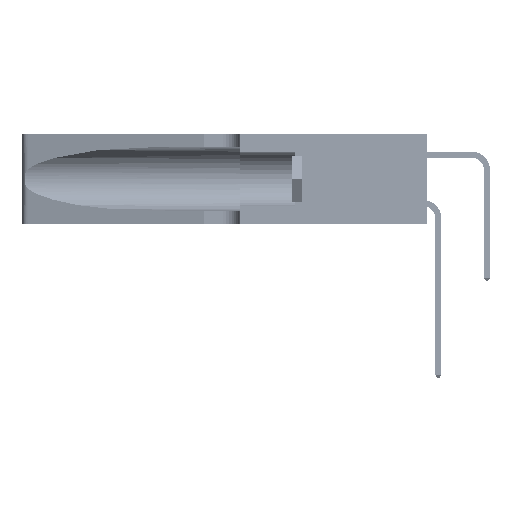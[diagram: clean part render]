
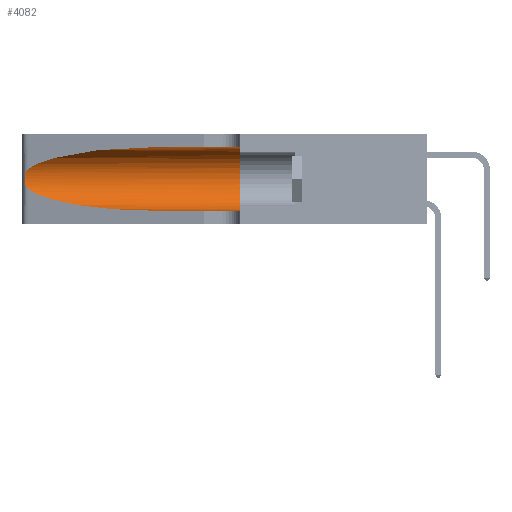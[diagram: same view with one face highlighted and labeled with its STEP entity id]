
A CAD part, left-side view. The second image highlights one B-rep face of the part: STEP entity #4082.
In plain terms, the highlighted cylindrical face has radius 3.308 mm (diameter 6.617 mm), a partial arc.
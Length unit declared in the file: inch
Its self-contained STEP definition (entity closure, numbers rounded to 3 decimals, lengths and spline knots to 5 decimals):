
#132 = LINE ( 'NONE', #53798, #2145 ) ;
#247 = CARTESIAN_POINT ( 'NONE',  ( 0.1305, 0.35, 0.185 ) ) ;
#2145 = VECTOR ( 'NONE', #22762, 39.37008 ) ;
#4082 = ADVANCED_FACE ( 'NONE', ( #48773 ), #19457, .F. ) ;
#4983 = VERTEX_POINT ( 'NONE', #8598 ) ;
#5031 = CIRCLE ( 'NONE', #31959, 0.13025 ) ;
#7638 = CARTESIAN_POINT ( 'NONE',  ( 0.25487, 1.22718, 0.22369 ) ) ;
#7841 = EDGE_CURVE ( 'NONE', #52570, #32961, #28715, .T. ) ;
#7964 = CARTESIAN_POINT ( 'NONE',  ( 0.1305, 0.72297, 0.05475 ) ) ;
#8035 = AXIS2_PLACEMENT_3D ( 'NONE', #45340, #50082, #14811 ) ;
#8598 = CARTESIAN_POINT ( 'NONE',  ( 0.1305, 0.35, 0.31525 ) ) ;
#8722 = CARTESIAN_POINT ( 'NONE',  ( 0.25789, 1.23486, 0.15765 ) ) ;
#9101 = CARTESIAN_POINT ( 'NONE',  ( 0.25555, 1.22994, 0.2215 ) ) ;
#11456 = ORIENTED_EDGE ( 'NONE', *, *, #47455, .F. ) ;
#12190 = CARTESIAN_POINT ( 'NONE',  ( 0.25487, 1.22718, 0.14631 ) ) ;
#13143 = CARTESIAN_POINT ( 'NONE',  ( 0.25555, 1.22993, 0.14849 ) ) ;
#14784 = CARTESIAN_POINT ( 'NONE',  ( 0.1305, 0.72297, 0.05475 ) ) ;
#14811 = DIRECTION ( 'NONE',  ( 0., 0., -1. ) ) ;
#16566 = CARTESIAN_POINT ( 'NONE',  ( 0.18966, 0.96281, 0.05475 ) ) ;
#17701 = CARTESIAN_POINT ( 'NONE',  ( 0.26018, 1.23835, 0.19895 ) ) ;
#18547 = ORIENTED_EDGE ( 'NONE', *, *, #20131, .F. ) ;
#19457 = CYLINDRICAL_SURFACE ( 'NONE', #8035, 0.13025 ) ;
#20131 = EDGE_CURVE ( 'NONE', #4983, #32767, #5031, .T. ) ;
#21354 = CARTESIAN_POINT ( 'NONE',  ( 0.26075, 1.23896, 0.178 ) ) ;
#21537 = CARTESIAN_POINT ( 'NONE',  ( 0.25487, 1.22718, 0.22369 ) ) ;
#22079 =( BOUNDED_CURVE ( )  B_SPLINE_CURVE ( 3, ( #42907, #56063, #25947, #7638 ),
 .UNSPECIFIED., .F., .F. ) 
 B_SPLINE_CURVE_WITH_KNOTS ( ( 4, 4 ),
 ( 1.5708, 2.84003 ),
 .UNSPECIFIED. ) 
 CURVE ( )  GEOMETRIC_REPRESENTATION_ITEM ( )  RATIONAL_B_SPLINE_CURVE ( ( 1., 0.87, 0.87, 1. ) ) 
 REPRESENTATION_ITEM ( '' )  );
#22762 = DIRECTION ( 'NONE',  ( 0., -1., 0. ) ) ;
#23532 = CARTESIAN_POINT ( 'NONE',  ( 0.25487, 1.22718, 0.22369 ) ) ;
#25947 = CARTESIAN_POINT ( 'NONE',  ( 0.2373, 1.15595, 0.28018 ) ) ;
#26295 = CARTESIAN_POINT ( 'NONE',  ( 0.25487, 1.22718, 0.14631 ) ) ;
#28172 = ORIENTED_EDGE ( 'NONE', *, *, #52831, .T. ) ;
#28715 = B_SPLINE_CURVE_WITH_KNOTS ( 'NONE', 3,
 ( #21537, #9101, #48048, #30320, #30687, #17701, #39070, #21354, #43444, #30505, #8722, #39252, #13143, #26295 ),
 .UNSPECIFIED., .F., .F.,
 ( 4, 2, 2, 2, 2, 2, 4 ),
 ( 0., 0.00027, 0.00053, 0.00107, 0.0016, 0.00187, 0.00214 ),
 .UNSPECIFIED. ) ;
#29254 = CARTESIAN_POINT ( 'NONE',  ( 0.1305, 0.35, 0.05475 ) ) ;
#29286 = LINE ( 'NONE', #52092, #39486 ) ;
#30225 = ORIENTED_EDGE ( 'NONE', *, *, #7841, .T. ) ;
#30320 = CARTESIAN_POINT ( 'NONE',  ( 0.25787, 1.23484, 0.2124 ) ) ;
#30505 = CARTESIAN_POINT ( 'NONE',  ( 0.25856, 1.23593, 0.16098 ) ) ;
#30687 = CARTESIAN_POINT ( 'NONE',  ( 0.25854, 1.2359, 0.20912 ) ) ;
#31304 = DIRECTION ( 'NONE',  ( 0., 0., 1. ) ) ;
#31565 = EDGE_CURVE ( 'NONE', #32961, #41404, #41634, .T. ) ;
#31959 = AXIS2_PLACEMENT_3D ( 'NONE', #247, #39860, #31304 ) ;
#32767 = VERTEX_POINT ( 'NONE', #29254 ) ;
#32961 = VERTEX_POINT ( 'NONE', #33638 ) ;
#33638 = CARTESIAN_POINT ( 'NONE',  ( 0.25487, 1.22718, 0.14631 ) ) ;
#36588 = VERTEX_POINT ( 'NONE', #53740 ) ;
#36699 = ORIENTED_EDGE ( 'NONE', *, *, #31565, .T. ) ;
#39070 = CARTESIAN_POINT ( 'NONE',  ( 0.26075, 1.23896, 0.19203 ) ) ;
#39252 = CARTESIAN_POINT ( 'NONE',  ( 0.25639, 1.23186, 0.15144 ) ) ;
#39486 = VECTOR ( 'NONE', #43495, 39.37008 ) ;
#39860 = DIRECTION ( 'NONE',  ( 0., 1., 0. ) ) ;
#41404 = VERTEX_POINT ( 'NONE', #14784 ) ;
#41517 = ORIENTED_EDGE ( 'NONE', *, *, #50818, .T. ) ;
#41634 =( BOUNDED_CURVE ( )  B_SPLINE_CURVE ( 3, ( #12190, #55650, #16566, #7964 ),
 .UNSPECIFIED., .F., .T. ) 
 B_SPLINE_CURVE_WITH_KNOTS ( ( 4, 4 ),
 ( 3.44316, 4.71239 ),
 .UNSPECIFIED. ) 
 CURVE ( )  GEOMETRIC_REPRESENTATION_ITEM ( )  RATIONAL_B_SPLINE_CURVE ( ( 1., 0.87, 0.87, 1. ) ) 
 REPRESENTATION_ITEM ( '' )  );
#42907 = CARTESIAN_POINT ( 'NONE',  ( 0.1305, 0.72297, 0.31525 ) ) ;
#43444 = CARTESIAN_POINT ( 'NONE',  ( 0.26017, 1.23833, 0.17102 ) ) ;
#43495 = DIRECTION ( 'NONE',  ( 0., -1., 0. ) ) ;
#45340 = CARTESIAN_POINT ( 'NONE',  ( 0.1305, 1.61858, 0.185 ) ) ;
#47455 = EDGE_CURVE ( 'NONE', #36588, #4983, #132, .T. ) ;
#48048 = CARTESIAN_POINT ( 'NONE',  ( 0.25639, 1.23184, 0.21858 ) ) ;
#48773 = FACE_OUTER_BOUND ( 'NONE', #50689, .T. ) ;
#50082 = DIRECTION ( 'NONE',  ( 0., -1., 0. ) ) ;
#50689 = EDGE_LOOP ( 'NONE', ( #28172, #30225, #36699, #41517, #18547, #11456 ) ) ;
#50818 = EDGE_CURVE ( 'NONE', #41404, #32767, #29286, .T. ) ;
#52092 = CARTESIAN_POINT ( 'NONE',  ( 0.1305, 1.61858, 0.05475 ) ) ;
#52570 = VERTEX_POINT ( 'NONE', #23532 ) ;
#52831 = EDGE_CURVE ( 'NONE', #36588, #52570, #22079, .T. ) ;
#53740 = CARTESIAN_POINT ( 'NONE',  ( 0.1305, 0.72297, 0.31525 ) ) ;
#53798 = CARTESIAN_POINT ( 'NONE',  ( 0.1305, 1.61858, 0.31525 ) ) ;
#55650 = CARTESIAN_POINT ( 'NONE',  ( 0.2373, 1.15595, 0.08982 ) ) ;
#56063 = CARTESIAN_POINT ( 'NONE',  ( 0.18966, 0.96281, 0.31525 ) ) ;
